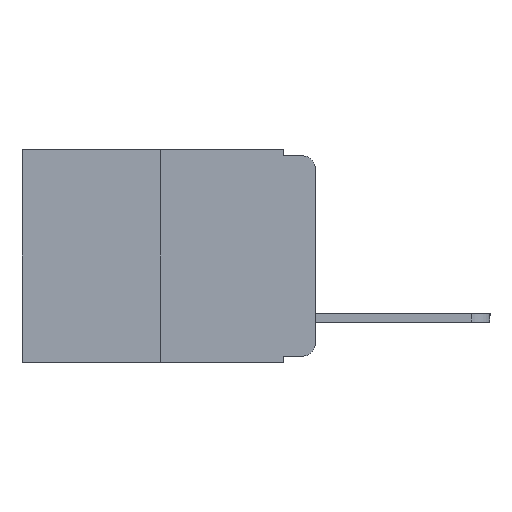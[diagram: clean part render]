
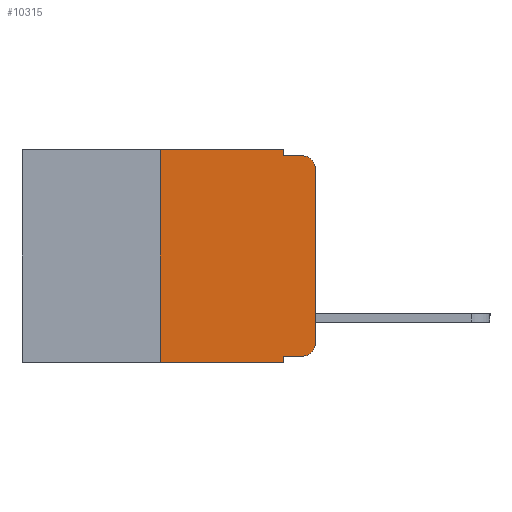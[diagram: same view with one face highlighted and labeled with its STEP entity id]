
A CAD part, left-side view. The second image highlights one B-rep face of the part: STEP entity #10315.
In plain terms, the highlighted planar face has unit normal (-1, 0, 0).
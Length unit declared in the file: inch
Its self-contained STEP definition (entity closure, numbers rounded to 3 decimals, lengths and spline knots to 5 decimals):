
#251 = FACE_OUTER_BOUND ( 'NONE', #10432, .T. ) ;
#444 = VERTEX_POINT ( 'NONE', #5431 ) ;
#475 = VERTEX_POINT ( 'NONE', #4130 ) ;
#526 = LINE ( 'NONE', #3930, #2357 ) ;
#534 = CARTESIAN_POINT ( 'NONE',  ( 0., 0., -0.313 ) ) ;
#927 = DIRECTION ( 'NONE',  ( -1., 0., 0. ) ) ;
#969 = EDGE_CURVE ( 'NONE', #1724, #475, #2265, .T. ) ;
#1079 = CIRCLE ( 'NONE', #6860, 0.02 ) ;
#1450 = EDGE_CURVE ( 'NONE', #475, #7360, #1690, .T. ) ;
#1489 = VERTEX_POINT ( 'NONE', #534 ) ;
#1690 = LINE ( 'NONE', #6755, #11021 ) ;
#1724 = VERTEX_POINT ( 'NONE', #8934 ) ;
#1728 = ORIENTED_EDGE ( 'NONE', *, *, #9406, .F. ) ;
#1876 = CARTESIAN_POINT ( 'NONE',  ( 0., 0.051, -0.333 ) ) ;
#2088 = VERTEX_POINT ( 'NONE', #2295 ) ;
#2132 = DIRECTION ( 'NONE',  ( 0., -1., 0. ) ) ;
#2179 = ORIENTED_EDGE ( 'NONE', *, *, #11117, .T. ) ;
#2265 = LINE ( 'NONE', #3774, #9218 ) ;
#2274 = EDGE_CURVE ( 'NONE', #11666, #1724, #10305, .T. ) ;
#2295 = CARTESIAN_POINT ( 'NONE',  ( 0., 0.051, -0.343 ) ) ;
#2305 = ORIENTED_EDGE ( 'NONE', *, *, #6884, .T. ) ;
#2357 = VECTOR ( 'NONE', #3010, 39.37008 ) ;
#2415 = AXIS2_PLACEMENT_3D ( 'NONE', #3376, #9708, #4305 ) ;
#2471 = ORIENTED_EDGE ( 'NONE', *, *, #8733, .F. ) ;
#3010 = DIRECTION ( 'NONE',  ( 0., -1., 0. ) ) ;
#3376 = CARTESIAN_POINT ( 'NONE',  ( 0., 0.473, 0. ) ) ;
#3411 = EDGE_CURVE ( 'NONE', #11363, #7688, #5659, .T. ) ;
#3493 = DIRECTION ( 'NONE',  ( -1., 0., 0. ) ) ;
#3774 = CARTESIAN_POINT ( 'NONE',  ( 0., 0.473, 0. ) ) ;
#3789 = DIRECTION ( 'NONE',  ( 0., -1., 0. ) ) ;
#3930 = CARTESIAN_POINT ( 'NONE',  ( 0., 0.051, -0.01 ) ) ;
#4071 = VECTOR ( 'NONE', #2132, 39.37008 ) ;
#4130 = CARTESIAN_POINT ( 'NONE',  ( 0., 0.051, 0. ) ) ;
#4305 = DIRECTION ( 'NONE',  ( 0., 0., -1. ) ) ;
#4924 = VECTOR ( 'NONE', #7610, 39.37008 ) ;
#5072 = VECTOR ( 'NONE', #7592, 39.37008 ) ;
#5092 = DIRECTION ( 'NONE',  ( 0., 0., 1. ) ) ;
#5182 = PLANE ( 'NONE',  #2415 ) ;
#5431 = CARTESIAN_POINT ( 'NONE',  ( 0., 0.02, -0.01 ) ) ;
#5500 = LINE ( 'NONE', #9404, #4924 ) ;
#5659 = LINE ( 'NONE', #1876, #5072 ) ;
#5713 = CARTESIAN_POINT ( 'NONE',  ( 0., 0.051, -0.333 ) ) ;
#6041 = CARTESIAN_POINT ( 'NONE',  ( 0., 0.25, 0. ) ) ;
#6170 = VERTEX_POINT ( 'NONE', #6637 ) ;
#6407 = CARTESIAN_POINT ( 'NONE',  ( 0., 0.02, -0.03 ) ) ;
#6604 = ORIENTED_EDGE ( 'NONE', *, *, #3411, .T. ) ;
#6637 = CARTESIAN_POINT ( 'NONE',  ( 0., 0., -0.03 ) ) ;
#6755 = CARTESIAN_POINT ( 'NONE',  ( 0., 0.051, 0. ) ) ;
#6860 = AXIS2_PLACEMENT_3D ( 'NONE', #6407, #927, #7286 ) ;
#6884 = EDGE_CURVE ( 'NONE', #11666, #2088, #9161, .T. ) ;
#7286 = DIRECTION ( 'NONE',  ( 0., 0., -1. ) ) ;
#7360 = VERTEX_POINT ( 'NONE', #10958 ) ;
#7592 = DIRECTION ( 'NONE',  ( 0., -1., 0. ) ) ;
#7610 = DIRECTION ( 'NONE',  ( 0., 0., -1. ) ) ;
#7619 = VECTOR ( 'NONE', #5092, 39.37008 ) ;
#7688 = VERTEX_POINT ( 'NONE', #7727 ) ;
#7727 = CARTESIAN_POINT ( 'NONE',  ( 0., 0.02, -0.333 ) ) ;
#7989 = ORIENTED_EDGE ( 'NONE', *, *, #969, .F. ) ;
#8000 = ORIENTED_EDGE ( 'NONE', *, *, #8510, .T. ) ;
#8432 = CARTESIAN_POINT ( 'NONE',  ( 0., 0.473, -0.343 ) ) ;
#8510 = EDGE_CURVE ( 'NONE', #6170, #444, #1079, .T. ) ;
#8733 = EDGE_CURVE ( 'NONE', #7360, #444, #526, .T. ) ;
#8898 = EDGE_CURVE ( 'NONE', #1489, #6170, #10007, .T. ) ;
#8925 = CARTESIAN_POINT ( 'NONE',  ( 0., 0.02, -0.313 ) ) ;
#8934 = CARTESIAN_POINT ( 'NONE',  ( 0., 0.25, 0. ) ) ;
#8947 = ORIENTED_EDGE ( 'NONE', *, *, #8898, .T. ) ;
#8956 = ORIENTED_EDGE ( 'NONE', *, *, #2274, .F. ) ;
#9161 = LINE ( 'NONE', #8432, #4071 ) ;
#9218 = VECTOR ( 'NONE', #3789, 39.37008 ) ;
#9404 = CARTESIAN_POINT ( 'NONE',  ( 0., 0.051, 0. ) ) ;
#9406 = EDGE_CURVE ( 'NONE', #11363, #2088, #5500, .T. ) ;
#9584 = CARTESIAN_POINT ( 'NONE',  ( 0., 0., 0. ) ) ;
#9708 = DIRECTION ( 'NONE',  ( 1., 0., 0. ) ) ;
#9732 = CARTESIAN_POINT ( 'NONE',  ( 0., 0.25, -0.343 ) ) ;
#9824 = DIRECTION ( 'NONE',  ( 0., 0., -1. ) ) ;
#9938 = ORIENTED_EDGE ( 'NONE', *, *, #1450, .F. ) ;
#10007 = LINE ( 'NONE', #9584, #7619 ) ;
#10031 = VECTOR ( 'NONE', #11380, 39.37008 ) ;
#10305 = LINE ( 'NONE', #6041, #10031 ) ;
#10315 = ADVANCED_FACE ( 'NONE', ( #251 ), #5182, .F. ) ;
#10432 = EDGE_LOOP ( 'NONE', ( #8947, #8000, #2471, #9938, #7989, #8956, #2305, #1728, #6604, #2179 ) ) ;
#10953 = CIRCLE ( 'NONE', #11656, 0.02 ) ;
#10958 = CARTESIAN_POINT ( 'NONE',  ( 0., 0.051, -0.01 ) ) ;
#11021 = VECTOR ( 'NONE', #11651, 39.37008 ) ;
#11117 = EDGE_CURVE ( 'NONE', #7688, #1489, #10953, .T. ) ;
#11363 = VERTEX_POINT ( 'NONE', #5713 ) ;
#11380 = DIRECTION ( 'NONE',  ( 0., 0., 1. ) ) ;
#11651 = DIRECTION ( 'NONE',  ( 0., 0., -1. ) ) ;
#11656 = AXIS2_PLACEMENT_3D ( 'NONE', #8925, #3493, #9824 ) ;
#11666 = VERTEX_POINT ( 'NONE', #9732 ) ;
